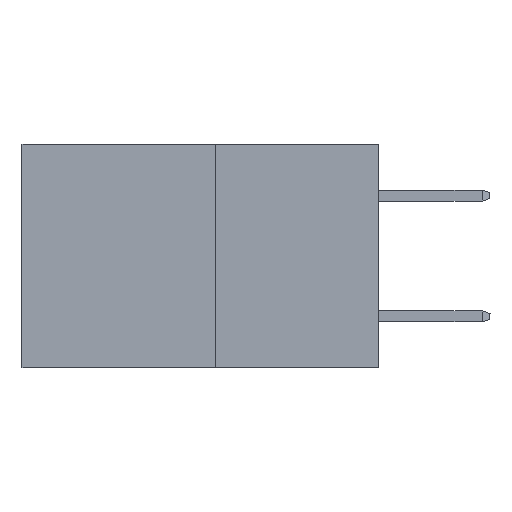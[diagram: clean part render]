
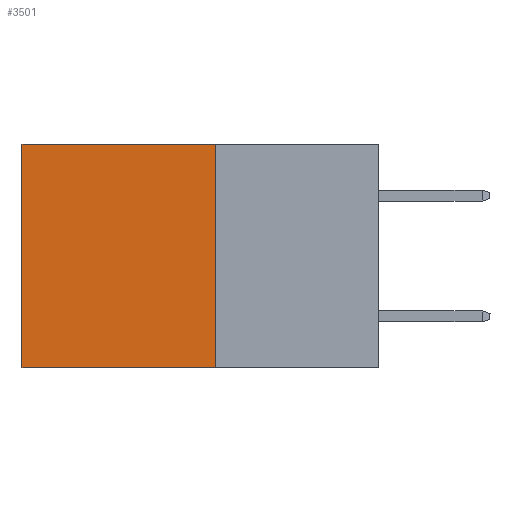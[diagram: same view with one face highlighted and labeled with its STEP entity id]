
A CAD part, left-side view. The second image highlights one B-rep face of the part: STEP entity #3501.
In plain terms, the highlighted planar face has unit normal (-1, 0, 0).
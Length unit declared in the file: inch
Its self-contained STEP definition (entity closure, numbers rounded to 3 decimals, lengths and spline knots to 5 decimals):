
#252 = LINE ( 'NONE', #3391, #8873 ) ;
#588 = DIRECTION ( 'NONE',  ( 0., 1., 0. ) ) ;
#608 = EDGE_CURVE ( 'NONE', #9504, #6838, #9666, .T. ) ;
#702 = EDGE_CURVE ( 'NONE', #3525, #6838, #252, .T. ) ;
#767 = CARTESIAN_POINT ( 'NONE',  ( 0.277, 0.27, 0. ) ) ;
#1038 = FACE_OUTER_BOUND ( 'NONE', #5031, .T. ) ;
#1193 = DIRECTION ( 'NONE',  ( 0., 1., 0. ) ) ;
#1401 = CARTESIAN_POINT ( 'NONE',  ( 0.277, 0.27, -0.37 ) ) ;
#1672 = CARTESIAN_POINT ( 'NONE',  ( 0.277, 0.59, -0.37 ) ) ;
#2081 = CARTESIAN_POINT ( 'NONE',  ( 0.277, 0.59, 0. ) ) ;
#2158 = EDGE_CURVE ( 'NONE', #9946, #9504, #8558, .T. ) ;
#3391 = CARTESIAN_POINT ( 'NONE',  ( 0.277, 0.59, -0.37 ) ) ;
#3460 = DIRECTION ( 'NONE',  ( 0., 0., -1. ) ) ;
#3501 = ADVANCED_FACE ( 'NONE', ( #1038 ), #3699, .F. ) ;
#3525 = VERTEX_POINT ( 'NONE', #2081 ) ;
#3601 = DIRECTION ( 'NONE',  ( 0., 0., -1. ) ) ;
#3639 = DIRECTION ( 'NONE',  ( 1., 0., 0. ) ) ;
#3656 = CARTESIAN_POINT ( 'NONE',  ( 0.277, 0.27, -0.37 ) ) ;
#3699 = PLANE ( 'NONE',  #8690 ) ;
#4020 = VECTOR ( 'NONE', #7621, 39.37008 ) ;
#4036 = CARTESIAN_POINT ( 'NONE',  ( 0.277, 0.27, -0.37 ) ) ;
#5031 = EDGE_LOOP ( 'NONE', ( #8493, #8969, #7892, #7631 ) ) ;
#5050 = VECTOR ( 'NONE', #588, 39.37008 ) ;
#5342 = EDGE_CURVE ( 'NONE', #9946, #3525, #9573, .T. ) ;
#6418 = CARTESIAN_POINT ( 'NONE',  ( 0.277, 0.27, -0.37 ) ) ;
#6838 = VERTEX_POINT ( 'NONE', #1672 ) ;
#7621 = DIRECTION ( 'NONE',  ( 0., 0., -1. ) ) ;
#7631 = ORIENTED_EDGE ( 'NONE', *, *, #5342, .T. ) ;
#7892 = ORIENTED_EDGE ( 'NONE', *, *, #2158, .F. ) ;
#8493 = ORIENTED_EDGE ( 'NONE', *, *, #702, .T. ) ;
#8558 = LINE ( 'NONE', #4036, #4020 ) ;
#8690 = AXIS2_PLACEMENT_3D ( 'NONE', #3656, #3639, #3601 ) ;
#8729 = CARTESIAN_POINT ( 'NONE',  ( 0.277, 0.27, 0. ) ) ;
#8873 = VECTOR ( 'NONE', #3460, 39.37008 ) ;
#8969 = ORIENTED_EDGE ( 'NONE', *, *, #608, .F. ) ;
#9504 = VERTEX_POINT ( 'NONE', #6418 ) ;
#9573 = LINE ( 'NONE', #767, #5050 ) ;
#9666 = LINE ( 'NONE', #1401, #10187 ) ;
#9946 = VERTEX_POINT ( 'NONE', #8729 ) ;
#10187 = VECTOR ( 'NONE', #1193, 39.37008 ) ;
